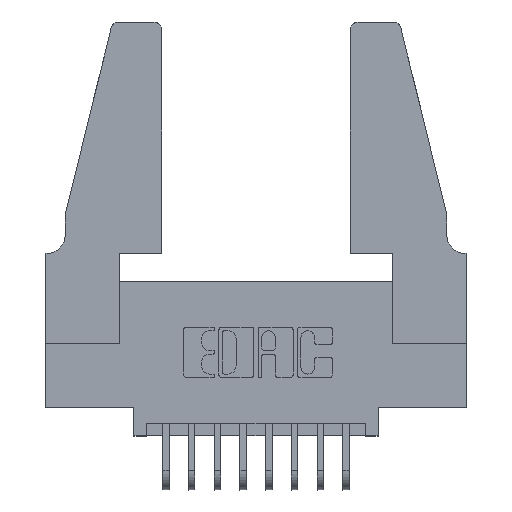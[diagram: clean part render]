
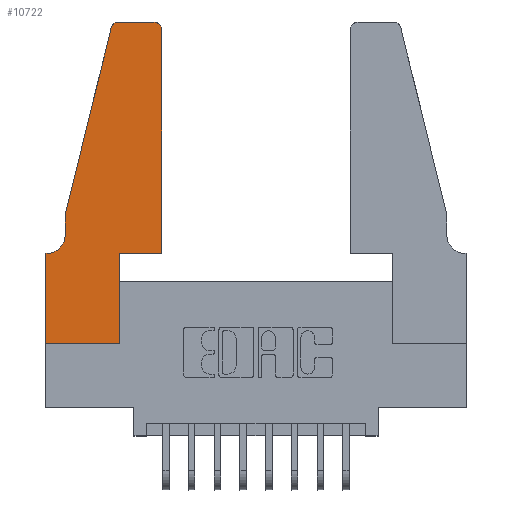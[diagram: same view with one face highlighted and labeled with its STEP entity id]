
A CAD part, top view. The second image highlights one B-rep face of the part: STEP entity #10722.
In plain terms, the highlighted planar face has unit normal (0, 0, 1).
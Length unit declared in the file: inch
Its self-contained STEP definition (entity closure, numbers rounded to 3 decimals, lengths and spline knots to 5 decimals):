
#325 = LINE ( 'NONE', #6520, #11914 ) ;
#357 = DIRECTION ( 'NONE',  ( 1., 0., 0. ) ) ;
#396 = VECTOR ( 'NONE', #5027, 39.37008 ) ;
#532 = ORIENTED_EDGE ( 'NONE', *, *, #966, .T. ) ;
#644 = ORIENTED_EDGE ( 'NONE', *, *, #4543, .T. ) ;
#771 = LINE ( 'NONE', #7624, #396 ) ;
#785 = LINE ( 'NONE', #6257, #14177 ) ;
#804 = CARTESIAN_POINT ( 'NONE',  ( 0.0755, 0.35, 0.37 ) ) ;
#931 = FACE_OUTER_BOUND ( 'NONE', #11659, .T. ) ;
#966 = EDGE_CURVE ( 'NONE', #3208, #11157, #785, .T. ) ;
#1073 = AXIS2_PLACEMENT_3D ( 'NONE', #1700, #1684, #1666 ) ;
#1202 = EDGE_CURVE ( 'NONE', #10900, #1603, #8422, .T. ) ;
#1603 = VERTEX_POINT ( 'NONE', #11060 ) ;
#1666 = DIRECTION ( 'NONE',  ( 1., 0., 0. ) ) ;
#1684 = DIRECTION ( 'NONE',  ( 0., 0., 1. ) ) ;
#1700 = CARTESIAN_POINT ( 'NONE',  ( 0.284, 1.22, 0.37 ) ) ;
#1845 = DIRECTION ( 'NONE',  ( 1., 0., 0. ) ) ;
#2008 = ORIENTED_EDGE ( 'NONE', *, *, #11913, .T. ) ;
#2212 = ORIENTED_EDGE ( 'NONE', *, *, #3510, .T. ) ;
#2617 = LINE ( 'NONE', #10575, #4563 ) ;
#2650 = ORIENTED_EDGE ( 'NONE', *, *, #10452, .T. ) ;
#2849 = EDGE_CURVE ( 'NONE', #10308, #3132, #4710, .T. ) ;
#3062 = DIRECTION ( 'NONE',  ( 0., 0., 1. ) ) ;
#3132 = VERTEX_POINT ( 'NONE', #6484 ) ;
#3190 = CIRCLE ( 'NONE', #1073, 0.03 ) ;
#3208 = VERTEX_POINT ( 'NONE', #4952 ) ;
#3276 = CARTESIAN_POINT ( 'NONE',  ( 0.25487, 1.22718, 0.37 ) ) ;
#3362 = CARTESIAN_POINT ( 'NONE',  ( 0.4205, 1.25, 0.37 ) ) ;
#3401 = ORIENTED_EDGE ( 'NONE', *, *, #2849, .T. ) ;
#3510 = EDGE_CURVE ( 'NONE', #12295, #10900, #3190, .T. ) ;
#3596 = LINE ( 'NONE', #804, #9407 ) ;
#4213 = VECTOR ( 'NONE', #357, 39.37008 ) ;
#4543 = EDGE_CURVE ( 'NONE', #11157, #4705, #13673, .T. ) ;
#4563 = VECTOR ( 'NONE', #7102, 39.37008 ) ;
#4705 = VERTEX_POINT ( 'NONE', #3362 ) ;
#4710 = CIRCLE ( 'NONE', #13431, 0.07 ) ;
#4952 = CARTESIAN_POINT ( 'NONE',  ( 0.4505, 0.35, 0.37 ) ) ;
#5027 = DIRECTION ( 'NONE',  ( 0., -1., 0. ) ) ;
#5031 = EDGE_CURVE ( 'NONE', #7743, #14775, #7320, .T. ) ;
#5989 = LINE ( 'NONE', #14117, #12091 ) ;
#6115 = ORIENTED_EDGE ( 'NONE', *, *, #1202, .T. ) ;
#6257 = CARTESIAN_POINT ( 'NONE',  ( 0.4505, 0.35, 0.37 ) ) ;
#6363 = ORIENTED_EDGE ( 'NONE', *, *, #7042, .T. ) ;
#6418 = PLANE ( 'NONE',  #10666 ) ;
#6422 = CARTESIAN_POINT ( 'NONE',  ( 0.2865, 0.35, 0.37 ) ) ;
#6484 = CARTESIAN_POINT ( 'NONE',  ( 0.0055, 0.35, 0.37 ) ) ;
#6520 = CARTESIAN_POINT ( 'NONE',  ( 0.2605, 1.25, 0.37 ) ) ;
#7042 = EDGE_CURVE ( 'NONE', #4705, #12295, #325, .T. ) ;
#7102 = DIRECTION ( 'NONE',  ( 0., 1., 0. ) ) ;
#7195 = CARTESIAN_POINT ( 'NONE',  ( 0.4505, 1.22, 0.37 ) ) ;
#7320 = LINE ( 'NONE', #10793, #4213 ) ;
#7624 = CARTESIAN_POINT ( 'NONE',  ( 0.0755, 0.5, 0.37 ) ) ;
#7743 = VERTEX_POINT ( 'NONE', #8939 ) ;
#7952 = ORIENTED_EDGE ( 'NONE', *, *, #5031, .T. ) ;
#8316 = ORIENTED_EDGE ( 'NONE', *, *, #10096, .T. ) ;
#8422 = LINE ( 'NONE', #14423, #11130 ) ;
#8716 = DIRECTION ( 'NONE',  ( 0., -1., 0. ) ) ;
#8802 = DIRECTION ( 'NONE',  ( 0., 0., 1. ) ) ;
#8920 = LINE ( 'NONE', #9833, #9290 ) ;
#8938 = ORIENTED_EDGE ( 'NONE', *, *, #11255, .T. ) ;
#8939 = CARTESIAN_POINT ( 'NONE',  ( 0., 0., 0.37 ) ) ;
#8955 = DIRECTION ( 'NONE',  ( -1., 0., 0. ) ) ;
#9027 = VERTEX_POINT ( 'NONE', #6422 ) ;
#9104 = ORIENTED_EDGE ( 'NONE', *, *, #9140, .T. ) ;
#9140 = EDGE_CURVE ( 'NONE', #3132, #12003, #3596, .T. ) ;
#9290 = VECTOR ( 'NONE', #8716, 39.37008 ) ;
#9407 = VECTOR ( 'NONE', #8955, 39.37008 ) ;
#9424 = CARTESIAN_POINT ( 'NONE',  ( 0.284, 1.25, 0.37 ) ) ;
#9833 = CARTESIAN_POINT ( 'NONE',  ( 0., 0., 0.37 ) ) ;
#9924 = CARTESIAN_POINT ( 'NONE',  ( 0., 0.35, 0.37 ) ) ;
#10001 = CARTESIAN_POINT ( 'NONE',  ( 0.4205, 1.22, 0.37 ) ) ;
#10064 = DIRECTION ( 'NONE',  ( -1., 0., 0. ) ) ;
#10096 = EDGE_CURVE ( 'NONE', #1603, #10308, #771, .T. ) ;
#10308 = VERTEX_POINT ( 'NONE', #12478 ) ;
#10349 = AXIS2_PLACEMENT_3D ( 'NONE', #10001, #3062, #11150 ) ;
#10452 = EDGE_CURVE ( 'NONE', #14775, #9027, #2617, .T. ) ;
#10575 = CARTESIAN_POINT ( 'NONE',  ( 0.2865, 0.35, 0.37 ) ) ;
#10666 = AXIS2_PLACEMENT_3D ( 'NONE', #9924, #8802, #1845 ) ;
#10722 = ADVANCED_FACE ( 'NONE', ( #931 ), #6418, .T. ) ;
#10793 = CARTESIAN_POINT ( 'NONE',  ( 0., 0., 0.37 ) ) ;
#10900 = VERTEX_POINT ( 'NONE', #3276 ) ;
#11060 = CARTESIAN_POINT ( 'NONE',  ( 0.0755, 0.5, 0.37 ) ) ;
#11130 = VECTOR ( 'NONE', #13400, 39.37008 ) ;
#11150 = DIRECTION ( 'NONE',  ( 1., 0., 0. ) ) ;
#11157 = VERTEX_POINT ( 'NONE', #7195 ) ;
#11176 = DIRECTION ( 'NONE',  ( -1., 0., 0. ) ) ;
#11192 = DIRECTION ( 'NONE',  ( 0., 0., -1. ) ) ;
#11255 = EDGE_CURVE ( 'NONE', #9027, #3208, #5989, .T. ) ;
#11304 = CARTESIAN_POINT ( 'NONE',  ( 0.0055, 0.42, 0.37 ) ) ;
#11588 = CARTESIAN_POINT ( 'NONE',  ( 0.2865, 0., 0.37 ) ) ;
#11659 = EDGE_LOOP ( 'NONE', ( #6363, #2212, #6115, #8316, #3401, #9104, #2008, #7952, #2650, #8938, #532, #644 ) ) ;
#11913 = EDGE_CURVE ( 'NONE', #12003, #7743, #8920, .T. ) ;
#11914 = VECTOR ( 'NONE', #10064, 39.37008 ) ;
#12003 = VERTEX_POINT ( 'NONE', #12238 ) ;
#12091 = VECTOR ( 'NONE', #13030, 39.37008 ) ;
#12238 = CARTESIAN_POINT ( 'NONE',  ( 0., 0.35, 0.37 ) ) ;
#12295 = VERTEX_POINT ( 'NONE', #9424 ) ;
#12478 = CARTESIAN_POINT ( 'NONE',  ( 0.0755, 0.42, 0.37 ) ) ;
#13030 = DIRECTION ( 'NONE',  ( 1., 0., 0. ) ) ;
#13400 = DIRECTION ( 'NONE',  ( -0.239, -0.971, 0. ) ) ;
#13431 = AXIS2_PLACEMENT_3D ( 'NONE', #11304, #11192, #11176 ) ;
#13673 = CIRCLE ( 'NONE', #10349, 0.03 ) ;
#14117 = CARTESIAN_POINT ( 'NONE',  ( 0.4505, 0.35, 0.37 ) ) ;
#14177 = VECTOR ( 'NONE', #14294, 39.37008 ) ;
#14294 = DIRECTION ( 'NONE',  ( 0., 1., 0. ) ) ;
#14423 = CARTESIAN_POINT ( 'NONE',  ( 0.0755, 0.5, 0.37 ) ) ;
#14775 = VERTEX_POINT ( 'NONE', #11588 ) ;
